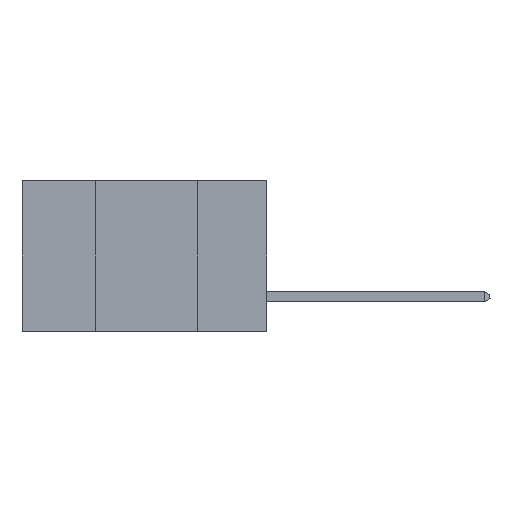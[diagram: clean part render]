
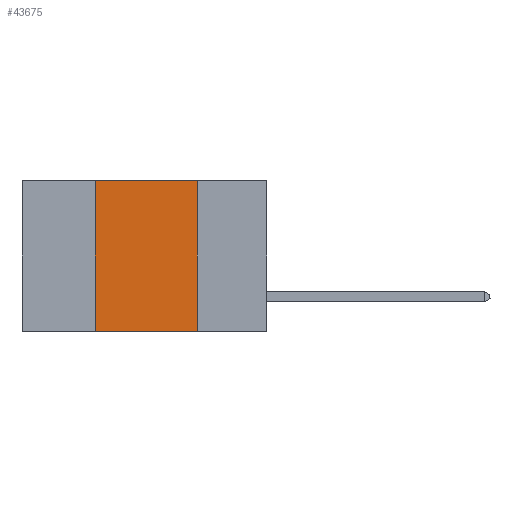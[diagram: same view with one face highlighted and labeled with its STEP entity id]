
A CAD part, left-side view. The second image highlights one B-rep face of the part: STEP entity #43675.
In plain terms, the highlighted planar face has unit normal (-1, 0, 0).
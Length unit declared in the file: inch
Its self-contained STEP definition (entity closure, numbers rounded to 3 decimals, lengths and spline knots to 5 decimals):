
#1018 = VERTEX_POINT ( 'NONE', #22978 ) ;
#3373 = ORIENTED_EDGE ( 'NONE', *, *, #42584, .F. ) ;
#3392 = CARTESIAN_POINT ( 'NONE',  ( 0., 0.6, 0. ) ) ;
#4950 = VERTEX_POINT ( 'NONE', #26306 ) ;
#6789 = ORIENTED_EDGE ( 'NONE', *, *, #22021, .F. ) ;
#9762 = CARTESIAN_POINT ( 'NONE',  ( 0., 0.42, -0.37 ) ) ;
#10394 = VECTOR ( 'NONE', #39596, 39.37008 ) ;
#10787 = CARTESIAN_POINT ( 'NONE',  ( 0., 0.6, -0.37 ) ) ;
#11124 = DIRECTION ( 'NONE',  ( 0., 0., -1. ) ) ;
#11356 = EDGE_CURVE ( 'NONE', #26860, #38467, #24230, .T. ) ;
#13070 = ORIENTED_EDGE ( 'NONE', *, *, #42900, .T. ) ;
#19438 = CARTESIAN_POINT ( 'NONE',  ( 0., 0.42, 0. ) ) ;
#20466 = EDGE_LOOP ( 'NONE', ( #3373, #6789, #20646, #13070 ) ) ;
#20646 = ORIENTED_EDGE ( 'NONE', *, *, #11356, .F. ) ;
#21673 = DIRECTION ( 'NONE',  ( 1., 0., 0. ) ) ;
#21746 = FACE_OUTER_BOUND ( 'NONE', #20466, .T. ) ;
#22021 = EDGE_CURVE ( 'NONE', #38467, #4950, #30992, .T. ) ;
#22950 = VECTOR ( 'NONE', #43698, 39.37008 ) ;
#22978 = CARTESIAN_POINT ( 'NONE',  ( 0., 0.17, -0.37 ) ) ;
#23161 = CARTESIAN_POINT ( 'NONE',  ( 0., 0.17, 0. ) ) ;
#23516 = LINE ( 'NONE', #23161, #22950 ) ;
#23641 = CARTESIAN_POINT ( 'NONE',  ( 0., 0.42, 0. ) ) ;
#24230 = LINE ( 'NONE', #19438, #10394 ) ;
#26306 = CARTESIAN_POINT ( 'NONE',  ( 0., 0.17, 0. ) ) ;
#26860 = VERTEX_POINT ( 'NONE', #9762 ) ;
#30232 = DIRECTION ( 'NONE',  ( 0., -1., 0. ) ) ;
#30992 = LINE ( 'NONE', #3392, #39539 ) ;
#31320 = AXIS2_PLACEMENT_3D ( 'NONE', #31431, #21673, #11124 ) ;
#31431 = CARTESIAN_POINT ( 'NONE',  ( 0., 0.6, 0. ) ) ;
#31569 = PLANE ( 'NONE',  #31320 ) ;
#36811 = LINE ( 'NONE', #10787, #43161 ) ;
#38467 = VERTEX_POINT ( 'NONE', #23641 ) ;
#39539 = VECTOR ( 'NONE', #30232, 39.37008 ) ;
#39596 = DIRECTION ( 'NONE',  ( 0., 0., 1. ) ) ;
#41631 = DIRECTION ( 'NONE',  ( 0., -1., 0. ) ) ;
#42584 = EDGE_CURVE ( 'NONE', #4950, #1018, #23516, .T. ) ;
#42900 = EDGE_CURVE ( 'NONE', #26860, #1018, #36811, .T. ) ;
#43161 = VECTOR ( 'NONE', #41631, 39.37008 ) ;
#43675 = ADVANCED_FACE ( 'NONE', ( #21746 ), #31569, .F. ) ;
#43698 = DIRECTION ( 'NONE',  ( 0., 0., -1. ) ) ;
